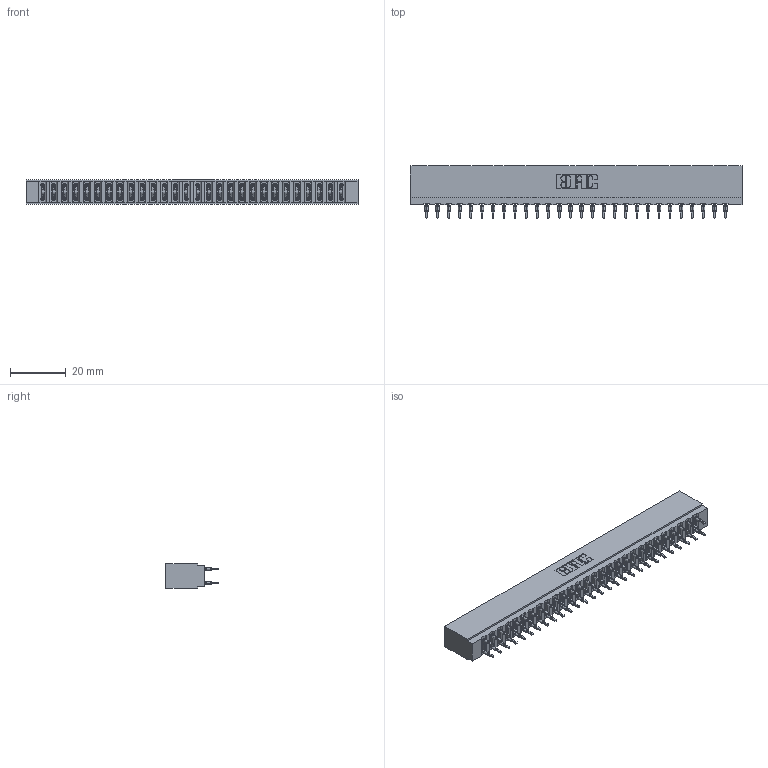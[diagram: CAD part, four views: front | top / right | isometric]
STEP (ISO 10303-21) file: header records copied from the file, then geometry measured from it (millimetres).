
FILE_DESCRIPTION (( 'STEP AP203' ), '1' );
FILE_NAME ('717-056-560-201.STEP', '2026-02-20T18:29:53', ( '' ), ( '' ), 'SwSTEP 2.0', 'SolidWorks 2023', '' );
FILE_SCHEMA (( 'CONFIG_CONTROL_DESIGN' ));
Length unit declared in the file: millimetre
Products named in the file (3): 745-292-001_560; 717-056-560-201; 717 Part_Insulator Option - 06
Assembly tree (57 placements, depth 2):
  717-056-560-201
    717 Part_Insulator Option - 06
    745-292-001_560  x56
Bounding box: 118.82 x 18.78 x 8.89 mm (x, y, z)
Volume: 10560.7 mm3; surface area: 16952.5 mm2
Topology: 57 solids, 57 shells, 5638 faces, 15427 edges, 9798 vertices
Faces by surface type: plane 2938, cylinder 1244, bspline 1120, torus 336
Entity records: 50228 total; most frequent: CARTESIAN_POINT 9227, ORIENTED_EDGE 8634, DIRECTION 7555, EDGE_CURVE 4317, VECTOR 3959, LINE 3959, VERTEX_POINT 2758, AXIS2_PLACEMENT_3D 1798
